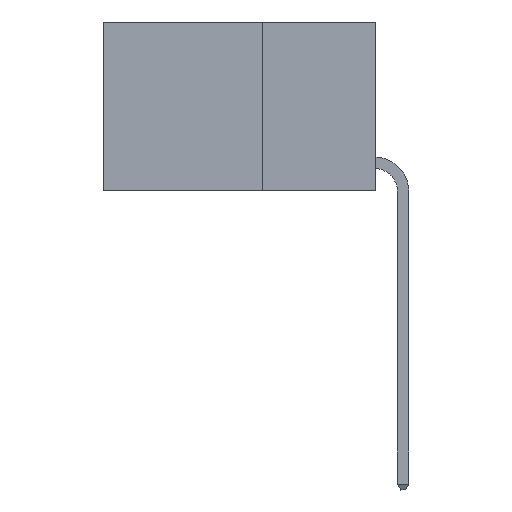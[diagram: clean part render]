
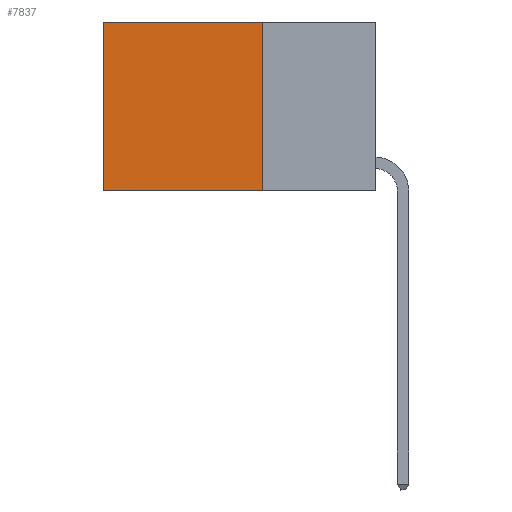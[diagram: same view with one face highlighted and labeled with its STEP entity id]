
A CAD part, left-side view. The second image highlights one B-rep face of the part: STEP entity #7837.
In plain terms, the highlighted planar face has unit normal (-1, 0, 0).
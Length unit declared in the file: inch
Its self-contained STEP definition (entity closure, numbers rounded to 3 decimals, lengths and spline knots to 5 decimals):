
#12 = VERTEX_POINT ( 'NONE', #5269 ) ;
#378 = VERTEX_POINT ( 'NONE', #11842 ) ;
#680 = VECTOR ( 'NONE', #9460, 39.37008 ) ;
#838 = LINE ( 'NONE', #9635, #680 ) ;
#955 = VERTEX_POINT ( 'NONE', #8303 ) ;
#1133 = ORIENTED_EDGE ( 'NONE', *, *, #5566, .F. ) ;
#1199 = LINE ( 'NONE', #4615, #12299 ) ;
#1434 = PLANE ( 'NONE',  #13487 ) ;
#1448 = FACE_OUTER_BOUND ( 'NONE', #3431, .T. ) ;
#1595 = ORIENTED_EDGE ( 'NONE', *, *, #10508, .F. ) ;
#2033 = LINE ( 'NONE', #5176, #2409 ) ;
#2187 = VECTOR ( 'NONE', #7437, 39.37008 ) ;
#2409 = VECTOR ( 'NONE', #4084, 39.37008 ) ;
#2717 = ORIENTED_EDGE ( 'NONE', *, *, #13148, .T. ) ;
#3080 = CARTESIAN_POINT ( 'NONE',  ( 0.2625, 0.6, 0. ) ) ;
#3354 = EDGE_CURVE ( 'NONE', #378, #13652, #838, .T. ) ;
#3431 = EDGE_LOOP ( 'NONE', ( #2717, #1595, #1133, #5781 ) ) ;
#4084 = DIRECTION ( 'NONE',  ( 0., 0., -1. ) ) ;
#4615 = CARTESIAN_POINT ( 'NONE',  ( 0.2625, 0.6, 0. ) ) ;
#5176 = CARTESIAN_POINT ( 'NONE',  ( 0.2625, 0.25, 0. ) ) ;
#5269 = CARTESIAN_POINT ( 'NONE',  ( 0.2625, 0.25, -0.37 ) ) ;
#5566 = EDGE_CURVE ( 'NONE', #378, #12, #2033, .T. ) ;
#5781 = ORIENTED_EDGE ( 'NONE', *, *, #3354, .T. ) ;
#5841 = DIRECTION ( 'NONE',  ( 1., 0., 0. ) ) ;
#6305 = CARTESIAN_POINT ( 'NONE',  ( 0.2625, 0.25, -0.37 ) ) ;
#7437 = DIRECTION ( 'NONE',  ( 0., 1., 0. ) ) ;
#7837 = ADVANCED_FACE ( 'NONE', ( #1448 ), #1434, .F. ) ;
#8303 = CARTESIAN_POINT ( 'NONE',  ( 0.2625, 0.6, -0.37 ) ) ;
#9460 = DIRECTION ( 'NONE',  ( 0., 1., 0. ) ) ;
#9635 = CARTESIAN_POINT ( 'NONE',  ( 0.2625, 0.25, 0. ) ) ;
#10508 = EDGE_CURVE ( 'NONE', #12, #955, #11647, .T. ) ;
#11647 = LINE ( 'NONE', #6305, #2187 ) ;
#11842 = CARTESIAN_POINT ( 'NONE',  ( 0.2625, 0.25, 0. ) ) ;
#12173 = CARTESIAN_POINT ( 'NONE',  ( 0.2625, 0.25, 0. ) ) ;
#12299 = VECTOR ( 'NONE', #13141, 39.37008 ) ;
#13141 = DIRECTION ( 'NONE',  ( 0., 0., -1. ) ) ;
#13148 = EDGE_CURVE ( 'NONE', #13652, #955, #1199, .T. ) ;
#13230 = DIRECTION ( 'NONE',  ( 0., 0., -1. ) ) ;
#13487 = AXIS2_PLACEMENT_3D ( 'NONE', #12173, #5841, #13230 ) ;
#13652 = VERTEX_POINT ( 'NONE', #3080 ) ;
